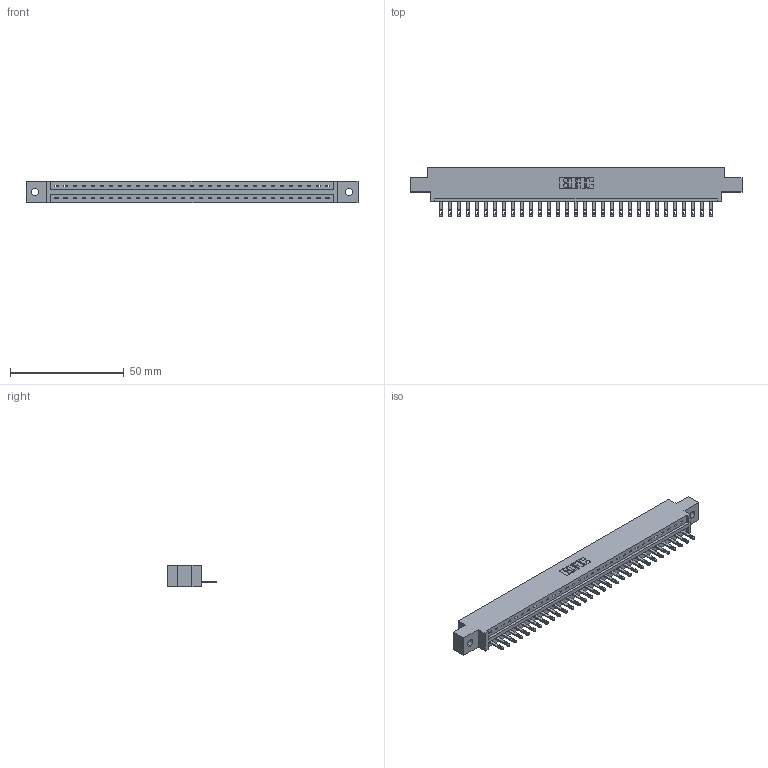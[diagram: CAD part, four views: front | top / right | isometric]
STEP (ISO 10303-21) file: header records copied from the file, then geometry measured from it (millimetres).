
FILE_DESCRIPTION (( 'STEP AP203' ), '1' );
FILE_NAME ('887-031-500-602.STEP', '2020-09-20T20:54:39', ( '' ), ( '' ), 'SwSTEP 2.0', 'SolidWorks 2020', '' );
FILE_SCHEMA (( 'CONFIG_CONTROL_DESIGN' ));
Length unit declared in the file: inch
Products named in the file (3): 345-292-001_345-293-100; 887-031-500-602; 837 Part_0.170 Offset - 0.128 Dia
Assembly tree (32 placements, depth 2):
  887-031-500-602
    837 Part_0.170 Offset - 0.128 Dia
    345-292-001_345-293-100  x31
Bounding box: 145.85 x 21.85 x 9.4 mm (x, y, z)
Volume: 14885.7 mm3; surface area: 15220 mm2
Topology: 32 solids, 32 shells, 1916 faces, 5903 edges, 3934 vertices
Faces by surface type: plane 1314, cylinder 602
Entity records: 24531 total; most frequent: CARTESIAN_POINT 4279, ORIENTED_EDGE 4246, DIRECTION 3625, EDGE_CURVE 2123, VECTOR 1991, LINE 1991, VERTEX_POINT 1414, AXIS2_PLACEMENT_3D 817
